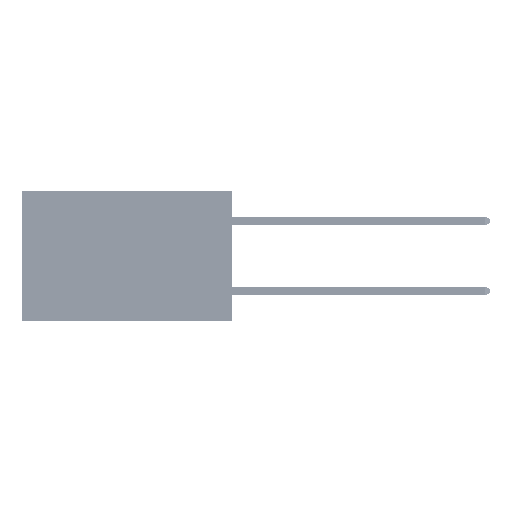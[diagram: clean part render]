
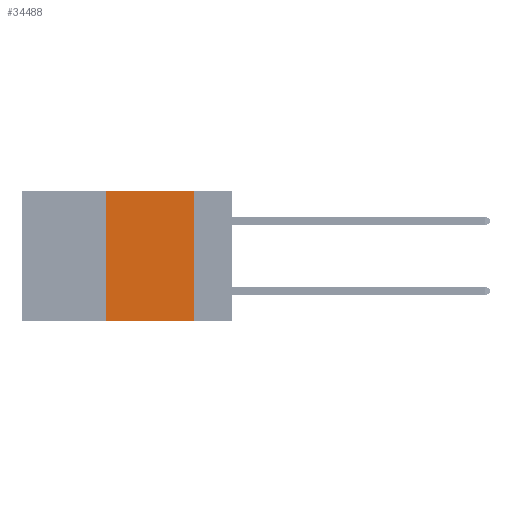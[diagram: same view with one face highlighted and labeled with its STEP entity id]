
A CAD part, left-side view. The second image highlights one B-rep face of the part: STEP entity #34488.
In plain terms, the highlighted planar face has unit normal (-1, 0, 0).
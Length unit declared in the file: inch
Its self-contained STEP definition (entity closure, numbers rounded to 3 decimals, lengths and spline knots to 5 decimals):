
#2268 = CARTESIAN_POINT ( 'NONE',  ( 0., 0.36, -0.37 ) ) ;
#4419 = DIRECTION ( 'NONE',  ( 1., 0., 0. ) ) ;
#4789 = CARTESIAN_POINT ( 'NONE',  ( 0., 0.11, 0. ) ) ;
#4931 = CARTESIAN_POINT ( 'NONE',  ( 0., 0.36, 0. ) ) ;
#4989 = EDGE_LOOP ( 'NONE', ( #27911, #39159, #36287, #23839 ) ) ;
#6062 = VERTEX_POINT ( 'NONE', #15170 ) ;
#7069 = CARTESIAN_POINT ( 'NONE',  ( 0., 0.6, 0. ) ) ;
#10919 = VERTEX_POINT ( 'NONE', #46116 ) ;
#11824 = EDGE_CURVE ( 'NONE', #32675, #10919, #39346, .T. ) ;
#13593 = EDGE_CURVE ( 'NONE', #46296, #6062, #17642, .T. ) ;
#15170 = CARTESIAN_POINT ( 'NONE',  ( 0., 0.11, -0.37 ) ) ;
#15470 = DIRECTION ( 'NONE',  ( 0., 0., 1. ) ) ;
#17450 = DIRECTION ( 'NONE',  ( 0., -1., 0. ) ) ;
#17642 = LINE ( 'NONE', #39060, #18537 ) ;
#18537 = VECTOR ( 'NONE', #38829, 39.37008 ) ;
#22333 = PLANE ( 'NONE',  #46056 ) ;
#23839 = ORIENTED_EDGE ( 'NONE', *, *, #13593, .T. ) ;
#26189 = VECTOR ( 'NONE', #30215, 39.37008 ) ;
#27911 = ORIENTED_EDGE ( 'NONE', *, *, #27992, .F. ) ;
#27992 = EDGE_CURVE ( 'NONE', #10919, #6062, #44147, .T. ) ;
#30215 = DIRECTION ( 'NONE',  ( 0., 0., -1. ) ) ;
#32675 = VERTEX_POINT ( 'NONE', #4931 ) ;
#33142 = DIRECTION ( 'NONE',  ( 0., 0., -1. ) ) ;
#34488 = ADVANCED_FACE ( 'NONE', ( #37142 ), #22333, .F. ) ;
#36165 = EDGE_CURVE ( 'NONE', #46296, #32675, #43730, .T. ) ;
#36287 = ORIENTED_EDGE ( 'NONE', *, *, #36165, .F. ) ;
#36367 = VECTOR ( 'NONE', #15470, 39.37008 ) ;
#36679 = CARTESIAN_POINT ( 'NONE',  ( 0., 0.6, 0. ) ) ;
#37101 = CARTESIAN_POINT ( 'NONE',  ( 0., 0.36, 0. ) ) ;
#37142 = FACE_OUTER_BOUND ( 'NONE', #4989, .T. ) ;
#38829 = DIRECTION ( 'NONE',  ( 0., -1., 0. ) ) ;
#39060 = CARTESIAN_POINT ( 'NONE',  ( 0., 0.6, -0.37 ) ) ;
#39159 = ORIENTED_EDGE ( 'NONE', *, *, #11824, .F. ) ;
#39346 = LINE ( 'NONE', #7069, #43198 ) ;
#43198 = VECTOR ( 'NONE', #17450, 39.37008 ) ;
#43730 = LINE ( 'NONE', #37101, #36367 ) ;
#44147 = LINE ( 'NONE', #4789, #26189 ) ;
#46056 = AXIS2_PLACEMENT_3D ( 'NONE', #36679, #4419, #33142 ) ;
#46116 = CARTESIAN_POINT ( 'NONE',  ( 0., 0.11, 0. ) ) ;
#46296 = VERTEX_POINT ( 'NONE', #2268 ) ;
